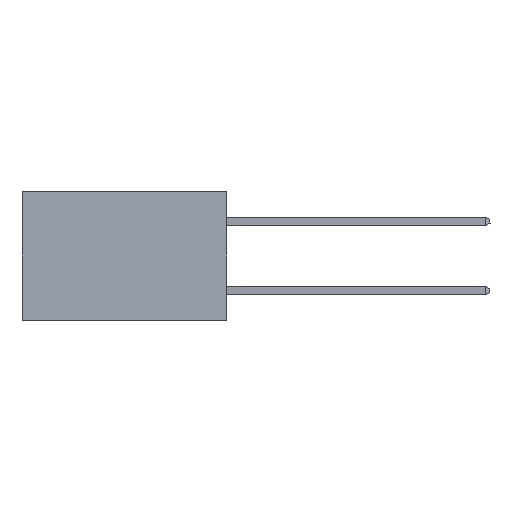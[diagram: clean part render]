
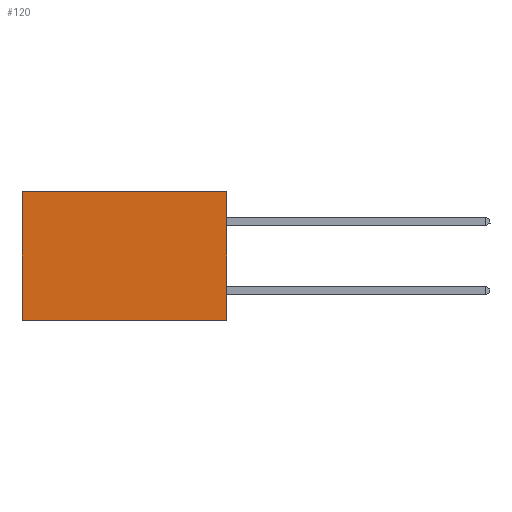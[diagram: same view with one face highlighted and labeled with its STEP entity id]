
A CAD part, left-side view. The second image highlights one B-rep face of the part: STEP entity #120.
In plain terms, the highlighted planar face has unit normal (-1, 0, 0).
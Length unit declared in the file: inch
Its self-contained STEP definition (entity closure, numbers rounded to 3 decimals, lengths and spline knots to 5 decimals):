
#15 = VERTEX_POINT ( 'NONE', #3969 ) ;
#120 = ADVANCED_FACE ( 'NONE', ( #7835 ), #4962, .F. ) ;
#767 = CARTESIAN_POINT ( 'NONE',  ( 0.277, 0., -0.37 ) ) ;
#886 = CARTESIAN_POINT ( 'NONE',  ( 0.277, 0.59, 0. ) ) ;
#953 = DIRECTION ( 'NONE',  ( 0., 0., -1. ) ) ;
#1284 = EDGE_CURVE ( 'NONE', #5841, #7845, #1903, .T. ) ;
#1316 = AXIS2_PLACEMENT_3D ( 'NONE', #8762, #9568, #6570 ) ;
#1576 = CARTESIAN_POINT ( 'NONE',  ( 0.277, 0.59, -0.37 ) ) ;
#1694 = LINE ( 'NONE', #9383, #7081 ) ;
#1903 = LINE ( 'NONE', #1576, #6011 ) ;
#2479 = DIRECTION ( 'NONE',  ( 0., 1., 0. ) ) ;
#2529 = CARTESIAN_POINT ( 'NONE',  ( 0.277, 0., 0. ) ) ;
#3619 = ORIENTED_EDGE ( 'NONE', *, *, #1284, .T. ) ;
#3649 = ORIENTED_EDGE ( 'NONE', *, *, #7651, .F. ) ;
#3729 = ORIENTED_EDGE ( 'NONE', *, *, #4557, .F. ) ;
#3738 = ORIENTED_EDGE ( 'NONE', *, *, #8723, .T. ) ;
#3969 = CARTESIAN_POINT ( 'NONE',  ( 0.277, 0., 0. ) ) ;
#4557 = EDGE_CURVE ( 'NONE', #15, #9667, #1694, .T. ) ;
#4962 = PLANE ( 'NONE',  #1316 ) ;
#5841 = VERTEX_POINT ( 'NONE', #886 ) ;
#6011 = VECTOR ( 'NONE', #953, 39.37008 ) ;
#6347 = VECTOR ( 'NONE', #9554, 39.37008 ) ;
#6570 = DIRECTION ( 'NONE',  ( 0., 0., -1. ) ) ;
#6731 = EDGE_LOOP ( 'NONE', ( #3619, #3649, #3729, #3738 ) ) ;
#7081 = VECTOR ( 'NONE', #9154, 39.37008 ) ;
#7588 = VECTOR ( 'NONE', #2479, 39.37008 ) ;
#7651 = EDGE_CURVE ( 'NONE', #9667, #7845, #8226, .T. ) ;
#7746 = CARTESIAN_POINT ( 'NONE',  ( 0.277, 0., -0.37 ) ) ;
#7835 = FACE_OUTER_BOUND ( 'NONE', #6731, .T. ) ;
#7845 = VERTEX_POINT ( 'NONE', #8513 ) ;
#8226 = LINE ( 'NONE', #7746, #6347 ) ;
#8513 = CARTESIAN_POINT ( 'NONE',  ( 0.277, 0.59, -0.37 ) ) ;
#8723 = EDGE_CURVE ( 'NONE', #15, #5841, #9362, .T. ) ;
#8762 = CARTESIAN_POINT ( 'NONE',  ( 0.277, 0., -0.37 ) ) ;
#9154 = DIRECTION ( 'NONE',  ( 0., 0., -1. ) ) ;
#9362 = LINE ( 'NONE', #2529, #7588 ) ;
#9383 = CARTESIAN_POINT ( 'NONE',  ( 0.277, 0., -0.37 ) ) ;
#9554 = DIRECTION ( 'NONE',  ( 0., 1., 0. ) ) ;
#9568 = DIRECTION ( 'NONE',  ( 1., 0., 0. ) ) ;
#9667 = VERTEX_POINT ( 'NONE', #767 ) ;
